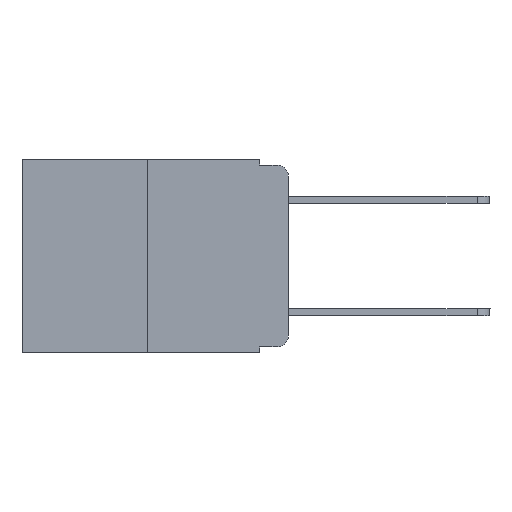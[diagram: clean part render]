
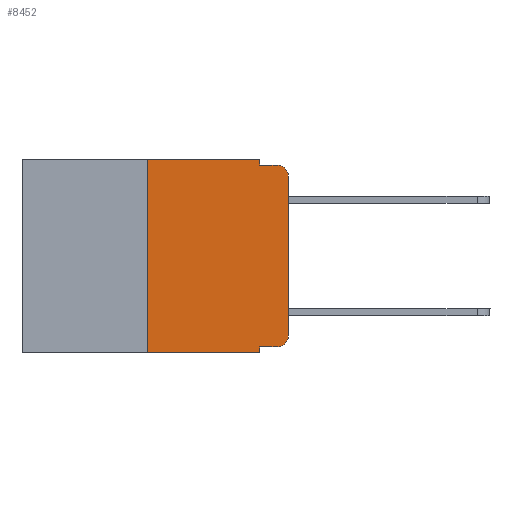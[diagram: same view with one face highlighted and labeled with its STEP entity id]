
A CAD part, left-side view. The second image highlights one B-rep face of the part: STEP entity #8452.
In plain terms, the highlighted planar face has unit normal (-1, 0, 0).
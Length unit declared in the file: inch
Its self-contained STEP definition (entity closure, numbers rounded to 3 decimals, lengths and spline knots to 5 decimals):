
#334 = VECTOR ( 'NONE', #791, 39.37008 ) ;
#354 = LINE ( 'NONE', #9810, #12773 ) ;
#558 = DIRECTION ( 'NONE',  ( 0., 0., 1. ) ) ;
#663 = VECTOR ( 'NONE', #2132, 39.37008 ) ;
#677 = CARTESIAN_POINT ( 'NONE',  ( 0., 0.473, 0. ) ) ;
#750 = LINE ( 'NONE', #4267, #12759 ) ;
#773 = VERTEX_POINT ( 'NONE', #11765 ) ;
#791 = DIRECTION ( 'NONE',  ( 0., -1., 0. ) ) ;
#971 = EDGE_CURVE ( 'NONE', #8478, #773, #750, .T. ) ;
#1376 = CIRCLE ( 'NONE', #3259, 0.02 ) ;
#1405 = VERTEX_POINT ( 'NONE', #13421 ) ;
#1906 = DIRECTION ( 'NONE',  ( 0., 0., -1. ) ) ;
#1933 = VERTEX_POINT ( 'NONE', #5252 ) ;
#2132 = DIRECTION ( 'NONE',  ( 0., -1., 0. ) ) ;
#2309 = VECTOR ( 'NONE', #11651, 39.37008 ) ;
#2460 = LINE ( 'NONE', #2954, #11074 ) ;
#2704 = ORIENTED_EDGE ( 'NONE', *, *, #971, .F. ) ;
#2891 = EDGE_CURVE ( 'NONE', #4821, #1405, #11732, .T. ) ;
#2954 = CARTESIAN_POINT ( 'NONE',  ( 0., 0.473, 0. ) ) ;
#3259 = AXIS2_PLACEMENT_3D ( 'NONE', #4079, #5634, #16584 ) ;
#3345 = EDGE_CURVE ( 'NONE', #7333, #4821, #354, .T. ) ;
#3451 = EDGE_CURVE ( 'NONE', #8992, #12055, #2460, .T. ) ;
#3720 = EDGE_CURVE ( 'NONE', #4517, #1405, #8034, .T. ) ;
#4079 = CARTESIAN_POINT ( 'NONE',  ( 0., 0.02, -0.313 ) ) ;
#4211 = DIRECTION ( 'NONE',  ( 0., 0., -1. ) ) ;
#4267 = CARTESIAN_POINT ( 'NONE',  ( 0., 0.051, 0. ) ) ;
#4517 = VERTEX_POINT ( 'NONE', #12072 ) ;
#4821 = VERTEX_POINT ( 'NONE', #6172 ) ;
#4943 = CARTESIAN_POINT ( 'NONE',  ( 0., 0.473, -0.343 ) ) ;
#5143 = DIRECTION ( 'NONE',  ( -1., 0., 0. ) ) ;
#5252 = CARTESIAN_POINT ( 'NONE',  ( 0., 0.02, -0.333 ) ) ;
#5341 = LINE ( 'NONE', #4943, #2309 ) ;
#5357 = AXIS2_PLACEMENT_3D ( 'NONE', #8168, #5143, #9578 ) ;
#5634 = DIRECTION ( 'NONE',  ( -1., 0., 0. ) ) ;
#6041 = CARTESIAN_POINT ( 'NONE',  ( 0., 0.051, 0. ) ) ;
#6172 = CARTESIAN_POINT ( 'NONE',  ( 0., 0., -0.03 ) ) ;
#6527 = EDGE_CURVE ( 'NONE', #8478, #1933, #15485, .T. ) ;
#6821 = ORIENTED_EDGE ( 'NONE', *, *, #3451, .F. ) ;
#6921 = LINE ( 'NONE', #14156, #14667 ) ;
#7270 = CARTESIAN_POINT ( 'NONE',  ( 0., 0.25, -0.343 ) ) ;
#7333 = VERTEX_POINT ( 'NONE', #16075 ) ;
#7557 = CARTESIAN_POINT ( 'NONE',  ( 0., 0.051, 0. ) ) ;
#7647 = CARTESIAN_POINT ( 'NONE',  ( 0., 0.051, -0.333 ) ) ;
#8034 = LINE ( 'NONE', #13376, #334 ) ;
#8145 = EDGE_CURVE ( 'NONE', #13054, #773, #5341, .T. ) ;
#8168 = CARTESIAN_POINT ( 'NONE',  ( 0., 0.02, -0.03 ) ) ;
#8236 = VECTOR ( 'NONE', #15804, 39.37008 ) ;
#8402 = DIRECTION ( 'NONE',  ( 0., -1., 0. ) ) ;
#8452 = ADVANCED_FACE ( 'NONE', ( #17391 ), #12965, .F. ) ;
#8478 = VERTEX_POINT ( 'NONE', #7647 ) ;
#8992 = VERTEX_POINT ( 'NONE', #10212 ) ;
#9578 = DIRECTION ( 'NONE',  ( 0., 0., -1. ) ) ;
#9810 = CARTESIAN_POINT ( 'NONE',  ( 0., 0., 0. ) ) ;
#10124 = DIRECTION ( 'NONE',  ( 1., 0., 0. ) ) ;
#10212 = CARTESIAN_POINT ( 'NONE',  ( 0., 0.25, 0. ) ) ;
#10306 = ORIENTED_EDGE ( 'NONE', *, *, #16167, .T. ) ;
#11074 = VECTOR ( 'NONE', #8402, 39.37008 ) ;
#11651 = DIRECTION ( 'NONE',  ( 0., -1., 0. ) ) ;
#11732 = CIRCLE ( 'NONE', #5357, 0.02 ) ;
#11765 = CARTESIAN_POINT ( 'NONE',  ( 0., 0.051, -0.343 ) ) ;
#11996 = ORIENTED_EDGE ( 'NONE', *, *, #3720, .F. ) ;
#12055 = VERTEX_POINT ( 'NONE', #7557 ) ;
#12072 = CARTESIAN_POINT ( 'NONE',  ( 0., 0.051, -0.01 ) ) ;
#12182 = ORIENTED_EDGE ( 'NONE', *, *, #14387, .F. ) ;
#12326 = ORIENTED_EDGE ( 'NONE', *, *, #3345, .T. ) ;
#12759 = VECTOR ( 'NONE', #4211, 39.37008 ) ;
#12773 = VECTOR ( 'NONE', #558, 39.37008 ) ;
#12965 = PLANE ( 'NONE',  #13292 ) ;
#13054 = VERTEX_POINT ( 'NONE', #7270 ) ;
#13292 = AXIS2_PLACEMENT_3D ( 'NONE', #677, #10124, #1906 ) ;
#13300 = EDGE_CURVE ( 'NONE', #12055, #4517, #14488, .T. ) ;
#13376 = CARTESIAN_POINT ( 'NONE',  ( 0., 0.051, -0.01 ) ) ;
#13421 = CARTESIAN_POINT ( 'NONE',  ( 0., 0.02, -0.01 ) ) ;
#13893 = ORIENTED_EDGE ( 'NONE', *, *, #6527, .T. ) ;
#13902 = ORIENTED_EDGE ( 'NONE', *, *, #8145, .T. ) ;
#14098 = DIRECTION ( 'NONE',  ( 0., 0., 1. ) ) ;
#14100 = CARTESIAN_POINT ( 'NONE',  ( 0., 0.051, -0.333 ) ) ;
#14156 = CARTESIAN_POINT ( 'NONE',  ( 0., 0.25, 0. ) ) ;
#14387 = EDGE_CURVE ( 'NONE', #13054, #8992, #6921, .T. ) ;
#14488 = LINE ( 'NONE', #6041, #8236 ) ;
#14667 = VECTOR ( 'NONE', #14098, 39.37008 ) ;
#14838 = ORIENTED_EDGE ( 'NONE', *, *, #13300, .F. ) ;
#15485 = LINE ( 'NONE', #14100, #663 ) ;
#15804 = DIRECTION ( 'NONE',  ( 0., 0., -1. ) ) ;
#15847 = ORIENTED_EDGE ( 'NONE', *, *, #2891, .T. ) ;
#16051 = EDGE_LOOP ( 'NONE', ( #12326, #15847, #11996, #14838, #6821, #12182, #13902, #2704, #13893, #10306 ) ) ;
#16075 = CARTESIAN_POINT ( 'NONE',  ( 0., 0., -0.313 ) ) ;
#16167 = EDGE_CURVE ( 'NONE', #1933, #7333, #1376, .T. ) ;
#16584 = DIRECTION ( 'NONE',  ( 0., 0., -1. ) ) ;
#17391 = FACE_OUTER_BOUND ( 'NONE', #16051, .T. ) ;
